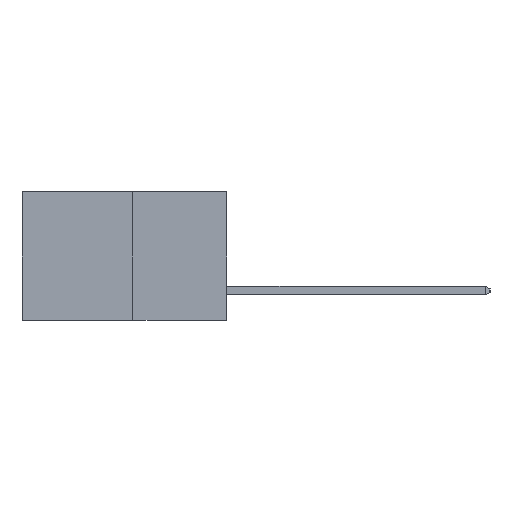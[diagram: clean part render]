
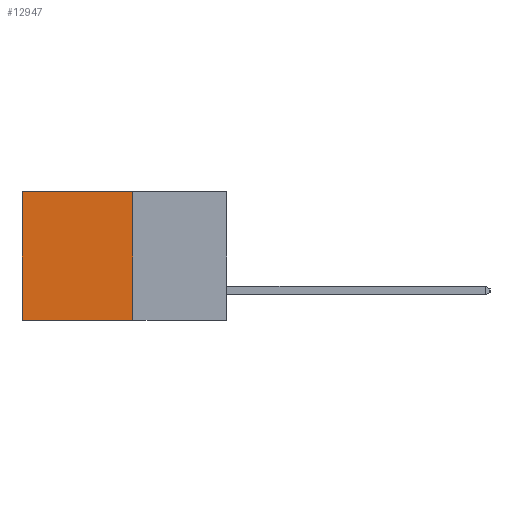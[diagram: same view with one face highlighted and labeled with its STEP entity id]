
A CAD part, left-side view. The second image highlights one B-rep face of the part: STEP entity #12947.
In plain terms, the highlighted planar face has unit normal (-1, 0, 0).
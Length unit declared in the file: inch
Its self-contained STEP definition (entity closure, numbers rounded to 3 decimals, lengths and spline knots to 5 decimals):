
#71 = CARTESIAN_POINT ( 'NONE',  ( 0.277, 0.59, -0.37 ) ) ;
#214 = CARTESIAN_POINT ( 'NONE',  ( 0.277, 0.59, -0.37 ) ) ;
#317 = EDGE_CURVE ( 'NONE', #1092, #8338, #9186, .T. ) ;
#603 = DIRECTION ( 'NONE',  ( 0., 0., -1. ) ) ;
#956 = EDGE_CURVE ( 'NONE', #1965, #1092, #9923, .T. ) ;
#1092 = VERTEX_POINT ( 'NONE', #6619 ) ;
#1965 = VERTEX_POINT ( 'NONE', #18758 ) ;
#4754 = DIRECTION ( 'NONE',  ( 0., 1., 0. ) ) ;
#4799 = CARTESIAN_POINT ( 'NONE',  ( 0.277, 0.27, -0.37 ) ) ;
#5040 = VECTOR ( 'NONE', #7648, 39.37008 ) ;
#5112 = DIRECTION ( 'NONE',  ( 0., 0., -1. ) ) ;
#5715 = ORIENTED_EDGE ( 'NONE', *, *, #16757, .F. ) ;
#5975 = VERTEX_POINT ( 'NONE', #7826 ) ;
#6284 = ORIENTED_EDGE ( 'NONE', *, *, #956, .T. ) ;
#6619 = CARTESIAN_POINT ( 'NONE',  ( 0.277, 0.59, 0. ) ) ;
#6706 = FACE_OUTER_BOUND ( 'NONE', #18458, .T. ) ;
#7648 = DIRECTION ( 'NONE',  ( 0., 1., 0. ) ) ;
#7826 = CARTESIAN_POINT ( 'NONE',  ( 0.277, 0.27, -0.37 ) ) ;
#8338 = VERTEX_POINT ( 'NONE', #214 ) ;
#8344 = CARTESIAN_POINT ( 'NONE',  ( 0.277, 0.27, -0.37 ) ) ;
#8938 = EDGE_CURVE ( 'NONE', #5975, #8338, #12113, .T. ) ;
#9022 = VECTOR ( 'NONE', #4754, 39.37008 ) ;
#9186 = LINE ( 'NONE', #71, #16831 ) ;
#9578 = CARTESIAN_POINT ( 'NONE',  ( 0.277, 0.27, -0.37 ) ) ;
#9923 = LINE ( 'NONE', #15385, #5040 ) ;
#11231 = DIRECTION ( 'NONE',  ( 0., 0., -1. ) ) ;
#11853 = ORIENTED_EDGE ( 'NONE', *, *, #8938, .F. ) ;
#12113 = LINE ( 'NONE', #4799, #9022 ) ;
#12947 = ADVANCED_FACE ( 'NONE', ( #6706 ), #19242, .F. ) ;
#13611 = ORIENTED_EDGE ( 'NONE', *, *, #317, .T. ) ;
#15385 = CARTESIAN_POINT ( 'NONE',  ( 0.277, 0.27, 0. ) ) ;
#16757 = EDGE_CURVE ( 'NONE', #1965, #5975, #19525, .T. ) ;
#16831 = VECTOR ( 'NONE', #603, 39.37008 ) ;
#18458 = EDGE_LOOP ( 'NONE', ( #13611, #11853, #5715, #6284 ) ) ;
#18493 = AXIS2_PLACEMENT_3D ( 'NONE', #9578, #20828, #11231 ) ;
#18758 = CARTESIAN_POINT ( 'NONE',  ( 0.277, 0.27, 0. ) ) ;
#19025 = VECTOR ( 'NONE', #5112, 39.37008 ) ;
#19242 = PLANE ( 'NONE',  #18493 ) ;
#19525 = LINE ( 'NONE', #8344, #19025 ) ;
#20828 = DIRECTION ( 'NONE',  ( 1., 0., 0. ) ) ;
